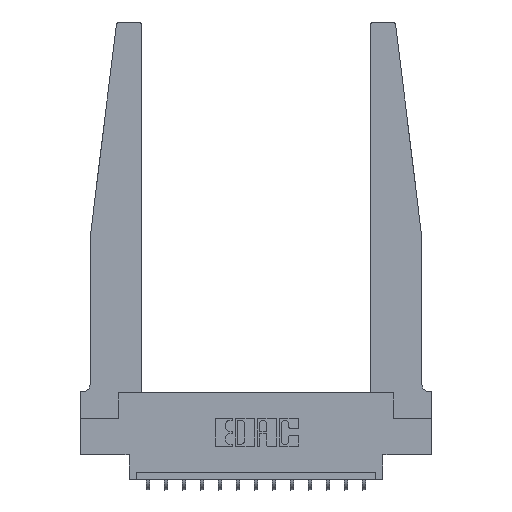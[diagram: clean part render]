
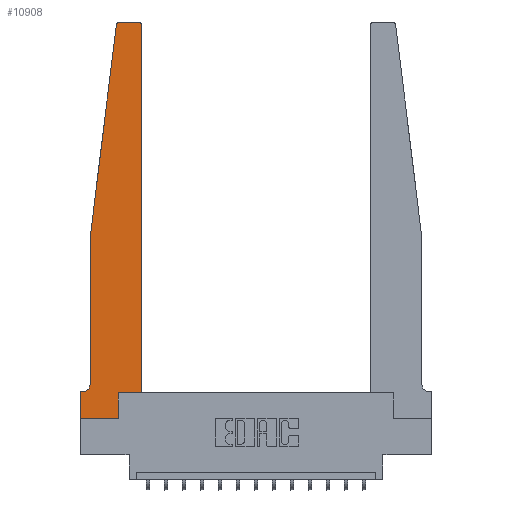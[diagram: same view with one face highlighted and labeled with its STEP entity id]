
A CAD part, top view. The second image highlights one B-rep face of the part: STEP entity #10908.
In plain terms, the highlighted planar face has unit normal (0, 0, 1).
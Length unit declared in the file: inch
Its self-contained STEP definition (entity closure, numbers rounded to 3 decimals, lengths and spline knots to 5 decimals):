
#106 = VERTEX_POINT ( 'NONE', #4486 ) ;
#237 = DIRECTION ( 'NONE',  ( 1., 0., 0. ) ) ;
#368 = DIRECTION ( 'NONE',  ( 0., -1., 0. ) ) ;
#566 = DIRECTION ( 'NONE',  ( 1., 0., 0. ) ) ;
#804 = DIRECTION ( 'NONE',  ( 0., 0., 1. ) ) ;
#1201 = DIRECTION ( 'NONE',  ( 0., 1., 0. ) ) ;
#1242 = CARTESIAN_POINT ( 'NONE',  ( 0.015, 0.2375, 0.37 ) ) ;
#1291 = CARTESIAN_POINT ( 'NONE',  ( 0.065, 1.25, 0.37 ) ) ;
#1348 = VECTOR ( 'NONE', #13679, 39.37008 ) ;
#1675 = EDGE_LOOP ( 'NONE', ( #8982, #7980, #11285, #16093, #11874, #6954, #15340, #8192, #16137, #6725, #5389, #9097 ) ) ;
#1933 = CARTESIAN_POINT ( 'NONE',  ( 0.065, 0.1875, 0.37 ) ) ;
#2186 = LINE ( 'NONE', #12751, #17158 ) ;
#2235 = EDGE_CURVE ( 'NONE', #5736, #16194, #15674, .T. ) ;
#2650 = CARTESIAN_POINT ( 'NONE',  ( 0.27653, 2.75, 0.37 ) ) ;
#2737 = VERTEX_POINT ( 'NONE', #3142 ) ;
#2738 = VERTEX_POINT ( 'NONE', #13482 ) ;
#3142 = CARTESIAN_POINT ( 'NONE',  ( 0.425, 2.72, 0.37 ) ) ;
#3212 = CARTESIAN_POINT ( 'NONE',  ( 0., 0.1875, 0.37 ) ) ;
#3257 = LINE ( 'NONE', #1933, #9246 ) ;
#3401 = VERTEX_POINT ( 'NONE', #15105 ) ;
#3953 = EDGE_CURVE ( 'NONE', #16194, #5488, #3257, .T. ) ;
#4206 = AXIS2_PLACEMENT_3D ( 'NONE', #1242, #9323, #6611 ) ;
#4343 = CARTESIAN_POINT ( 'NONE',  ( 0.25, 2.75, 0.37 ) ) ;
#4486 = CARTESIAN_POINT ( 'NONE',  ( 0.065, 1.25, 0.37 ) ) ;
#4611 = EDGE_CURVE ( 'NONE', #106, #5736, #16646, .T. ) ;
#5138 = AXIS2_PLACEMENT_3D ( 'NONE', #3212, #804, #14135 ) ;
#5147 = DIRECTION ( 'NONE',  ( 0., 0., 1. ) ) ;
#5241 = EDGE_CURVE ( 'NONE', #5488, #3401, #2186, .T. ) ;
#5358 = DIRECTION ( 'NONE',  ( -0.122, -0.992, 0. ) ) ;
#5389 = ORIENTED_EDGE ( 'NONE', *, *, #14834, .T. ) ;
#5455 = LINE ( 'NONE', #12298, #1348 ) ;
#5488 = VERTEX_POINT ( 'NONE', #15246 ) ;
#5736 = VERTEX_POINT ( 'NONE', #12095 ) ;
#5927 = FACE_OUTER_BOUND ( 'NONE', #1675, .T. ) ;
#6611 = DIRECTION ( 'NONE',  ( -1., 0., 0. ) ) ;
#6659 = LINE ( 'NONE', #12369, #7775 ) ;
#6725 = ORIENTED_EDGE ( 'NONE', *, *, #13469, .T. ) ;
#6954 = ORIENTED_EDGE ( 'NONE', *, *, #3953, .T. ) ;
#6975 = VERTEX_POINT ( 'NONE', #7852 ) ;
#7138 = PLANE ( 'NONE',  #5138 ) ;
#7266 = DIRECTION ( 'NONE',  ( -1., 0., 0. ) ) ;
#7323 = CIRCLE ( 'NONE', #15746, 0.03 ) ;
#7482 = VECTOR ( 'NONE', #17029, 39.37008 ) ;
#7532 = DIRECTION ( 'NONE',  ( 0., -1., 0. ) ) ;
#7775 = VECTOR ( 'NONE', #237, 39.37008 ) ;
#7852 = CARTESIAN_POINT ( 'NONE',  ( 0.2605, 0.18, 0.37 ) ) ;
#7879 = CIRCLE ( 'NONE', #11848, 0.03 ) ;
#7963 = LINE ( 'NONE', #1291, #15497 ) ;
#7980 = ORIENTED_EDGE ( 'NONE', *, *, #15542, .T. ) ;
#8104 = VERTEX_POINT ( 'NONE', #8474 ) ;
#8192 = ORIENTED_EDGE ( 'NONE', *, *, #13069, .T. ) ;
#8474 = CARTESIAN_POINT ( 'NONE',  ( 0.395, 2.75, 0.37 ) ) ;
#8982 = ORIENTED_EDGE ( 'NONE', *, *, #10357, .T. ) ;
#9056 = VERTEX_POINT ( 'NONE', #17395 ) ;
#9097 = ORIENTED_EDGE ( 'NONE', *, *, #15775, .T. ) ;
#9246 = VECTOR ( 'NONE', #7266, 39.37008 ) ;
#9323 = DIRECTION ( 'NONE',  ( 0., 0., -1. ) ) ;
#9750 = CARTESIAN_POINT ( 'NONE',  ( 0.015, 0.1875, 0.37 ) ) ;
#10172 = CARTESIAN_POINT ( 'NONE',  ( 0.24675, 2.72367, 0.37 ) ) ;
#10204 = VERTEX_POINT ( 'NONE', #2650 ) ;
#10330 = LINE ( 'NONE', #11768, #10680 ) ;
#10357 = EDGE_CURVE ( 'NONE', #8104, #10204, #16533, .T. ) ;
#10484 = CARTESIAN_POINT ( 'NONE',  ( 0.425, 0.18, 0.37 ) ) ;
#10644 = EDGE_CURVE ( 'NONE', #16378, #106, #7963, .T. ) ;
#10680 = VECTOR ( 'NONE', #1201, 39.37008 ) ;
#10908 = ADVANCED_FACE ( 'NONE', ( #5927 ), #7138, .T. ) ;
#11285 = ORIENTED_EDGE ( 'NONE', *, *, #10644, .T. ) ;
#11523 = EDGE_CURVE ( 'NONE', #9056, #6975, #5455, .T. ) ;
#11768 = CARTESIAN_POINT ( 'NONE',  ( 0.425, 0.18, 0.37 ) ) ;
#11837 = LINE ( 'NONE', #10484, #7482 ) ;
#11848 = AXIS2_PLACEMENT_3D ( 'NONE', #12250, #5147, #15851 ) ;
#11874 = ORIENTED_EDGE ( 'NONE', *, *, #2235, .T. ) ;
#12095 = CARTESIAN_POINT ( 'NONE',  ( 0.065, 0.2375, 0.37 ) ) ;
#12250 = CARTESIAN_POINT ( 'NONE',  ( 0.395, 2.72, 0.37 ) ) ;
#12298 = CARTESIAN_POINT ( 'NONE',  ( 0.2605, 0.18, 0.37 ) ) ;
#12369 = CARTESIAN_POINT ( 'NONE',  ( 0., 0., 0.37 ) ) ;
#12406 = VECTOR ( 'NONE', #15007, 39.37008 ) ;
#12621 = DIRECTION ( 'NONE',  ( 0., 0., 1. ) ) ;
#12751 = CARTESIAN_POINT ( 'NONE',  ( 0., 0., 0.37 ) ) ;
#12922 = VECTOR ( 'NONE', #368, 39.37008 ) ;
#13069 = EDGE_CURVE ( 'NONE', #3401, #9056, #6659, .T. ) ;
#13469 = EDGE_CURVE ( 'NONE', #6975, #2738, #11837, .T. ) ;
#13482 = CARTESIAN_POINT ( 'NONE',  ( 0.425, 0.18, 0.37 ) ) ;
#13679 = DIRECTION ( 'NONE',  ( 0., 1., 0. ) ) ;
#13906 = CARTESIAN_POINT ( 'NONE',  ( 0.27653, 2.72, 0.37 ) ) ;
#14135 = DIRECTION ( 'NONE',  ( 1., 0., 0. ) ) ;
#14834 = EDGE_CURVE ( 'NONE', #2738, #2737, #10330, .T. ) ;
#15007 = DIRECTION ( 'NONE',  ( -1., 0., 0. ) ) ;
#15105 = CARTESIAN_POINT ( 'NONE',  ( 0., 0., 0.37 ) ) ;
#15190 = CARTESIAN_POINT ( 'NONE',  ( 0.065, 1.25, 0.37 ) ) ;
#15246 = CARTESIAN_POINT ( 'NONE',  ( 0., 0.1875, 0.37 ) ) ;
#15340 = ORIENTED_EDGE ( 'NONE', *, *, #5241, .T. ) ;
#15497 = VECTOR ( 'NONE', #5358, 39.37008 ) ;
#15542 = EDGE_CURVE ( 'NONE', #10204, #16378, #7323, .T. ) ;
#15674 = CIRCLE ( 'NONE', #4206, 0.05 ) ;
#15746 = AXIS2_PLACEMENT_3D ( 'NONE', #13906, #12621, #566 ) ;
#15775 = EDGE_CURVE ( 'NONE', #2737, #8104, #7879, .T. ) ;
#15851 = DIRECTION ( 'NONE',  ( 1., 0., 0. ) ) ;
#16093 = ORIENTED_EDGE ( 'NONE', *, *, #4611, .T. ) ;
#16137 = ORIENTED_EDGE ( 'NONE', *, *, #11523, .T. ) ;
#16194 = VERTEX_POINT ( 'NONE', #9750 ) ;
#16378 = VERTEX_POINT ( 'NONE', #10172 ) ;
#16533 = LINE ( 'NONE', #4343, #12406 ) ;
#16646 = LINE ( 'NONE', #15190, #12922 ) ;
#17029 = DIRECTION ( 'NONE',  ( 1., 0., 0. ) ) ;
#17158 = VECTOR ( 'NONE', #7532, 39.37008 ) ;
#17395 = CARTESIAN_POINT ( 'NONE',  ( 0.2605, 0., 0.37 ) ) ;
